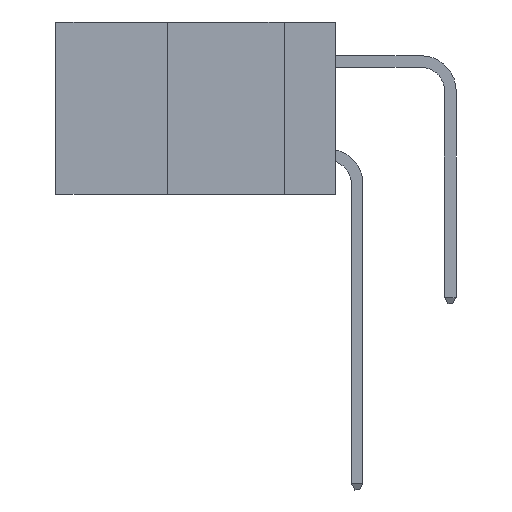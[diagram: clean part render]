
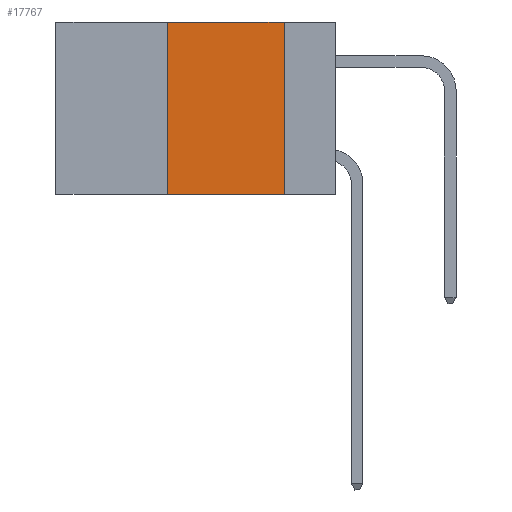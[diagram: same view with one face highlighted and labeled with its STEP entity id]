
A CAD part, left-side view. The second image highlights one B-rep face of the part: STEP entity #17767.
In plain terms, the highlighted planar face has unit normal (-1, 0, 0).
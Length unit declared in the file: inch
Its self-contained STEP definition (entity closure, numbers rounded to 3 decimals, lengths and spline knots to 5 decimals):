
#40 = DIRECTION ( 'NONE',  ( 0., 0., -1. ) ) ;
#180 = VERTEX_POINT ( 'NONE', #19643 ) ;
#515 = LINE ( 'NONE', #11509, #2188 ) ;
#699 = CARTESIAN_POINT ( 'NONE',  ( 0., 0.6, -0.37 ) ) ;
#2188 = VECTOR ( 'NONE', #15010, 39.37008 ) ;
#3157 = CARTESIAN_POINT ( 'NONE',  ( 0., 0.11, -0.37 ) ) ;
#3412 = DIRECTION ( 'NONE',  ( 0., 0., 1. ) ) ;
#3571 = EDGE_CURVE ( 'NONE', #4903, #3650, #6817, .T. ) ;
#3650 = VERTEX_POINT ( 'NONE', #3157 ) ;
#3706 = VECTOR ( 'NONE', #13710, 39.37008 ) ;
#4903 = VERTEX_POINT ( 'NONE', #13568 ) ;
#5602 = DIRECTION ( 'NONE',  ( 1., 0., 0. ) ) ;
#5759 = VECTOR ( 'NONE', #15260, 39.37008 ) ;
#6600 = EDGE_CURVE ( 'NONE', #9174, #4903, #515, .T. ) ;
#6817 = LINE ( 'NONE', #18938, #3706 ) ;
#6884 = EDGE_LOOP ( 'NONE', ( #8375, #18693, #22419, #16379 ) ) ;
#7691 = LINE ( 'NONE', #699, #5759 ) ;
#8375 = ORIENTED_EDGE ( 'NONE', *, *, #3571, .F. ) ;
#9174 = VERTEX_POINT ( 'NONE', #11493 ) ;
#9417 = EDGE_CURVE ( 'NONE', #180, #9174, #21602, .T. ) ;
#9976 = FACE_OUTER_BOUND ( 'NONE', #6884, .T. ) ;
#11493 = CARTESIAN_POINT ( 'NONE',  ( 0., 0.36, 0. ) ) ;
#11509 = CARTESIAN_POINT ( 'NONE',  ( 0., 0.6, 0. ) ) ;
#13568 = CARTESIAN_POINT ( 'NONE',  ( 0., 0.11, 0. ) ) ;
#13710 = DIRECTION ( 'NONE',  ( 0., 0., -1. ) ) ;
#13790 = CARTESIAN_POINT ( 'NONE',  ( 0., 0.36, 0. ) ) ;
#15010 = DIRECTION ( 'NONE',  ( 0., -1., 0. ) ) ;
#15260 = DIRECTION ( 'NONE',  ( 0., -1., 0. ) ) ;
#16379 = ORIENTED_EDGE ( 'NONE', *, *, #18772, .T. ) ;
#17721 = CARTESIAN_POINT ( 'NONE',  ( 0., 0.6, 0. ) ) ;
#17767 = ADVANCED_FACE ( 'NONE', ( #9976 ), #21467, .F. ) ;
#18693 = ORIENTED_EDGE ( 'NONE', *, *, #6600, .F. ) ;
#18772 = EDGE_CURVE ( 'NONE', #180, #3650, #7691, .T. ) ;
#18938 = CARTESIAN_POINT ( 'NONE',  ( 0., 0.11, 0. ) ) ;
#19364 = AXIS2_PLACEMENT_3D ( 'NONE', #17721, #5602, #40 ) ;
#19643 = CARTESIAN_POINT ( 'NONE',  ( 0., 0.36, -0.37 ) ) ;
#21467 = PLANE ( 'NONE',  #19364 ) ;
#21602 = LINE ( 'NONE', #13790, #22428 ) ;
#22419 = ORIENTED_EDGE ( 'NONE', *, *, #9417, .F. ) ;
#22428 = VECTOR ( 'NONE', #3412, 39.37008 ) ;
